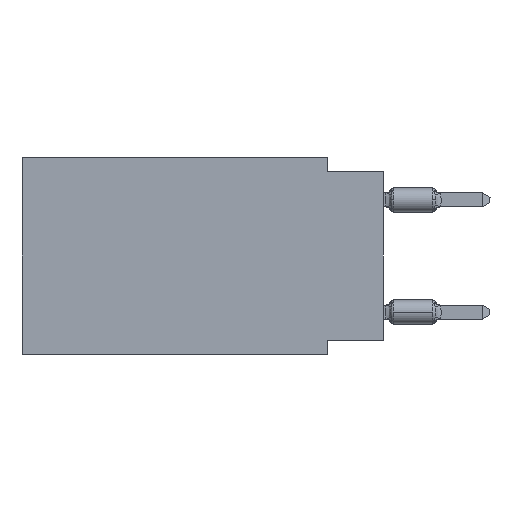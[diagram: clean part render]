
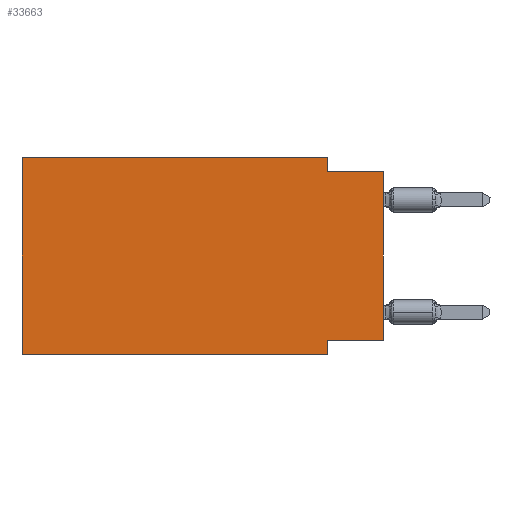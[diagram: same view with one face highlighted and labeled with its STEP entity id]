
A CAD part, left-side view. The second image highlights one B-rep face of the part: STEP entity #33663.
In plain terms, the highlighted planar face has unit normal (-1, 0, 0).
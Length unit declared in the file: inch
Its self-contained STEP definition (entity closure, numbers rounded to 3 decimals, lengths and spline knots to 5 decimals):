
#23 = ORIENTED_EDGE ( 'NONE', *, *, #3130, .F. ) ;
#708 = CARTESIAN_POINT ( 'NONE',  ( 0., 0.645, -0.35 ) ) ;
#1784 = EDGE_CURVE ( 'NONE', #31193, #38914, #34337, .T. ) ;
#1945 = DIRECTION ( 'NONE',  ( 0., -1., 0. ) ) ;
#2733 = VECTOR ( 'NONE', #12756, 39.37008 ) ;
#3130 = EDGE_CURVE ( 'NONE', #38914, #32930, #26528, .T. ) ;
#3407 = VERTEX_POINT ( 'NONE', #12177 ) ;
#4168 = LINE ( 'NONE', #21626, #31749 ) ;
#5011 = VERTEX_POINT ( 'NONE', #33135 ) ;
#5331 = VECTOR ( 'NONE', #1945, 39.37008 ) ;
#5605 = ORIENTED_EDGE ( 'NONE', *, *, #1784, .F. ) ;
#8295 = DIRECTION ( 'NONE',  ( 0., -1., 0. ) ) ;
#8877 = ORIENTED_EDGE ( 'NONE', *, *, #29222, .T. ) ;
#9210 = LINE ( 'NONE', #21821, #46586 ) ;
#9462 = EDGE_CURVE ( 'NONE', #29331, #17715, #33411, .T. ) ;
#11955 = CARTESIAN_POINT ( 'NONE',  ( 0., 0.645, -0.35 ) ) ;
#12177 = CARTESIAN_POINT ( 'NONE',  ( 0., 0., -0.325 ) ) ;
#12756 = DIRECTION ( 'NONE',  ( 0., 0., 1. ) ) ;
#13481 = DIRECTION ( 'NONE',  ( 0., 1., 0. ) ) ;
#13806 = DIRECTION ( 'NONE',  ( 0., -1., 0. ) ) ;
#16146 = LINE ( 'NONE', #33593, #48195 ) ;
#17715 = VERTEX_POINT ( 'NONE', #50115 ) ;
#17725 = ORIENTED_EDGE ( 'NONE', *, *, #52389, .F. ) ;
#21337 = PLANE ( 'NONE',  #38693 ) ;
#21626 = CARTESIAN_POINT ( 'NONE',  ( 0., 0.1, -0.35 ) ) ;
#21627 = ORIENTED_EDGE ( 'NONE', *, *, #26059, .F. ) ;
#21821 = CARTESIAN_POINT ( 'NONE',  ( 0., 0., -0.025 ) ) ;
#22181 = DIRECTION ( 'NONE',  ( 0., 0., -1. ) ) ;
#22877 = CARTESIAN_POINT ( 'NONE',  ( 0., 0.1, -0.025 ) ) ;
#24147 = ORIENTED_EDGE ( 'NONE', *, *, #24568, .F. ) ;
#24568 = EDGE_CURVE ( 'NONE', #42465, #17715, #4168, .T. ) ;
#24799 = EDGE_LOOP ( 'NONE', ( #8877, #44491, #23, #5605, #21627, #50684, #24147, #17725 ) ) ;
#25629 = LINE ( 'NONE', #25918, #2733 ) ;
#25845 = VECTOR ( 'NONE', #8295, 39.37008 ) ;
#25918 = CARTESIAN_POINT ( 'NONE',  ( 0., 0., 0. ) ) ;
#26059 = EDGE_CURVE ( 'NONE', #29331, #31193, #16146, .T. ) ;
#26528 = LINE ( 'NONE', #44281, #32139 ) ;
#29222 = EDGE_CURVE ( 'NONE', #3407, #5011, #25629, .T. ) ;
#29331 = VERTEX_POINT ( 'NONE', #708 ) ;
#30476 = FACE_OUTER_BOUND ( 'NONE', #24799, .T. ) ;
#31193 = VERTEX_POINT ( 'NONE', #48104 ) ;
#31749 = VECTOR ( 'NONE', #39080, 39.37008 ) ;
#32139 = VECTOR ( 'NONE', #56055, 39.37008 ) ;
#32930 = VERTEX_POINT ( 'NONE', #22877 ) ;
#33135 = CARTESIAN_POINT ( 'NONE',  ( 0., 0., -0.025 ) ) ;
#33411 = LINE ( 'NONE', #11955, #5331 ) ;
#33593 = CARTESIAN_POINT ( 'NONE',  ( 0., 0.645, 0. ) ) ;
#33663 = ADVANCED_FACE ( 'NONE', ( #30476 ), #21337, .F. ) ;
#34337 = LINE ( 'NONE', #51813, #25845 ) ;
#35499 = LINE ( 'NONE', #49249, #46788 ) ;
#38511 = CARTESIAN_POINT ( 'NONE',  ( 0., 0.645, 0. ) ) ;
#38693 = AXIS2_PLACEMENT_3D ( 'NONE', #38511, #55995, #22181 ) ;
#38914 = VERTEX_POINT ( 'NONE', #39661 ) ;
#39080 = DIRECTION ( 'NONE',  ( 0., 0., -1. ) ) ;
#39661 = CARTESIAN_POINT ( 'NONE',  ( 0., 0.1, 0. ) ) ;
#42465 = VERTEX_POINT ( 'NONE', #53971 ) ;
#44281 = CARTESIAN_POINT ( 'NONE',  ( 0., 0.1, 0. ) ) ;
#44491 = ORIENTED_EDGE ( 'NONE', *, *, #48413, .F. ) ;
#46586 = VECTOR ( 'NONE', #13806, 39.37008 ) ;
#46788 = VECTOR ( 'NONE', #13481, 39.37008 ) ;
#48104 = CARTESIAN_POINT ( 'NONE',  ( 0., 0.645, 0. ) ) ;
#48189 = DIRECTION ( 'NONE',  ( 0., 0., 1. ) ) ;
#48195 = VECTOR ( 'NONE', #48189, 39.37008 ) ;
#48413 = EDGE_CURVE ( 'NONE', #32930, #5011, #9210, .T. ) ;
#49249 = CARTESIAN_POINT ( 'NONE',  ( 0., 0., -0.325 ) ) ;
#50115 = CARTESIAN_POINT ( 'NONE',  ( 0., 0.1, -0.35 ) ) ;
#50684 = ORIENTED_EDGE ( 'NONE', *, *, #9462, .T. ) ;
#51813 = CARTESIAN_POINT ( 'NONE',  ( 0., 0.645, 0. ) ) ;
#52389 = EDGE_CURVE ( 'NONE', #3407, #42465, #35499, .T. ) ;
#53971 = CARTESIAN_POINT ( 'NONE',  ( 0., 0.1, -0.325 ) ) ;
#55995 = DIRECTION ( 'NONE',  ( 1., 0., 0. ) ) ;
#56055 = DIRECTION ( 'NONE',  ( 0., 0., -1. ) ) ;
